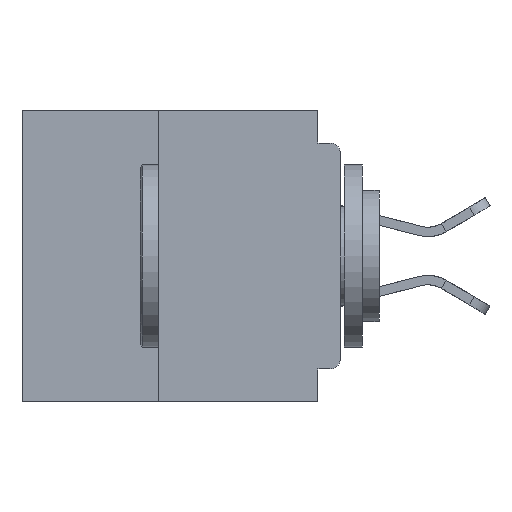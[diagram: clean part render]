
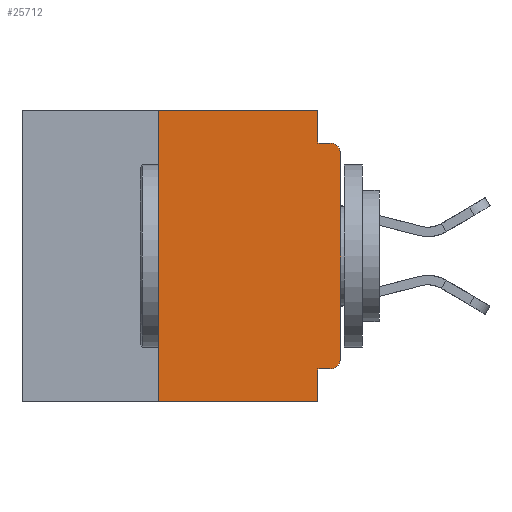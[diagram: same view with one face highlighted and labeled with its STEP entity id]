
A CAD part, left-side view. The second image highlights one B-rep face of the part: STEP entity #25712.
In plain terms, the highlighted planar face has unit normal (-1, 0, 0).
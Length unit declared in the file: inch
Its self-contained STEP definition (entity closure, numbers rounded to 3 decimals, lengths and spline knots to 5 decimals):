
#529 = DIRECTION ( 'NONE',  ( 0., 0., 1. ) ) ;
#967 = CARTESIAN_POINT ( 'NONE',  ( 0., 0.015, -0.355 ) ) ;
#1643 = VERTEX_POINT ( 'NONE', #35151 ) ;
#2192 = DIRECTION ( 'NONE',  ( 0., -1., 0. ) ) ;
#2508 = CIRCLE ( 'NONE', #37248, 0.015 ) ;
#2940 = CARTESIAN_POINT ( 'NONE',  ( 0., 0., -0.355 ) ) ;
#3272 = VECTOR ( 'NONE', #37952, 39.37008 ) ;
#4359 = VERTEX_POINT ( 'NONE', #12154 ) ;
#4495 = CARTESIAN_POINT ( 'NONE',  ( 0., 0.015, -0.34 ) ) ;
#5583 = VECTOR ( 'NONE', #36931, 39.37008 ) ;
#5776 = ORIENTED_EDGE ( 'NONE', *, *, #41378, .T. ) ;
#5811 = DIRECTION ( 'NONE',  ( 0., 0., -1. ) ) ;
#6164 = VERTEX_POINT ( 'NONE', #18352 ) ;
#6285 = LINE ( 'NONE', #29455, #47510 ) ;
#8066 = CARTESIAN_POINT ( 'NONE',  ( 0., 0.031, -0.4 ) ) ;
#8406 = DIRECTION ( 'NONE',  ( 0., 0., -1. ) ) ;
#11451 = EDGE_CURVE ( 'NONE', #26773, #46012, #16477, .T. ) ;
#11455 = AXIS2_PLACEMENT_3D ( 'NONE', #20209, #35841, #12506 ) ;
#11961 = ORIENTED_EDGE ( 'NONE', *, *, #47953, .T. ) ;
#12154 = CARTESIAN_POINT ( 'NONE',  ( 0., 0.015, -0.045 ) ) ;
#12506 = DIRECTION ( 'NONE',  ( 0., 0., -1. ) ) ;
#12715 = VECTOR ( 'NONE', #5811, 39.37008 ) ;
#13444 = EDGE_CURVE ( 'NONE', #37648, #26773, #26313, .T. ) ;
#13562 = LINE ( 'NONE', #2940, #3272 ) ;
#15649 = LINE ( 'NONE', #8066, #36321 ) ;
#16477 = LINE ( 'NONE', #44474, #46131 ) ;
#16908 = ORIENTED_EDGE ( 'NONE', *, *, #21993, .F. ) ;
#16915 = ORIENTED_EDGE ( 'NONE', *, *, #31370, .F. ) ;
#17288 = CARTESIAN_POINT ( 'NONE',  ( 0., 0.25, 0. ) ) ;
#17357 = DIRECTION ( 'NONE',  ( -1., 0., 0. ) ) ;
#18352 = CARTESIAN_POINT ( 'NONE',  ( 0., 0., -0.34 ) ) ;
#18478 = CARTESIAN_POINT ( 'NONE',  ( 0., 0.437, -0.4 ) ) ;
#20209 = CARTESIAN_POINT ( 'NONE',  ( 0., 0.437, 0. ) ) ;
#20778 = ORIENTED_EDGE ( 'NONE', *, *, #11451, .F. ) ;
#21427 = VECTOR ( 'NONE', #529, 39.37008 ) ;
#21993 = EDGE_CURVE ( 'NONE', #46012, #23897, #33446, .T. ) ;
#22427 = DIRECTION ( 'NONE',  ( 0., -1., 0. ) ) ;
#22482 = VERTEX_POINT ( 'NONE', #967 ) ;
#22801 = EDGE_CURVE ( 'NONE', #37648, #30056, #34600, .T. ) ;
#23517 = EDGE_CURVE ( 'NONE', #1643, #4359, #46537, .T. ) ;
#23897 = VERTEX_POINT ( 'NONE', #27563 ) ;
#24270 = VECTOR ( 'NONE', #22427, 39.37008 ) ;
#24434 = CARTESIAN_POINT ( 'NONE',  ( 0., 0.031, -0.355 ) ) ;
#25228 = CARTESIAN_POINT ( 'NONE',  ( 0., 0.031, 0. ) ) ;
#25274 = DIRECTION ( 'NONE',  ( 0., -1., 0. ) ) ;
#25410 = CARTESIAN_POINT ( 'NONE',  ( 0., 0.25, -0.4 ) ) ;
#25712 = ADVANCED_FACE ( 'NONE', ( #36022 ), #31965, .F. ) ;
#26313 = LINE ( 'NONE', #44622, #5583 ) ;
#26773 = VERTEX_POINT ( 'NONE', #17288 ) ;
#27563 = CARTESIAN_POINT ( 'NONE',  ( 0., 0.031, -0.045 ) ) ;
#27802 = CARTESIAN_POINT ( 'NONE',  ( 0., 0., 0. ) ) ;
#29455 = CARTESIAN_POINT ( 'NONE',  ( 0., 0., -0.045 ) ) ;
#30056 = VERTEX_POINT ( 'NONE', #31667 ) ;
#31370 = EDGE_CURVE ( 'NONE', #49707, #30056, #15649, .T. ) ;
#31377 = ORIENTED_EDGE ( 'NONE', *, *, #22801, .T. ) ;
#31667 = CARTESIAN_POINT ( 'NONE',  ( 0., 0.031, -0.4 ) ) ;
#31727 = DIRECTION ( 'NONE',  ( -1., 0., 0. ) ) ;
#31965 = PLANE ( 'NONE',  #11455 ) ;
#32606 = CARTESIAN_POINT ( 'NONE',  ( 0., 0.031, 0. ) ) ;
#33248 = AXIS2_PLACEMENT_3D ( 'NONE', #40561, #17357, #44407 ) ;
#33367 = EDGE_CURVE ( 'NONE', #22482, #49707, #13562, .T. ) ;
#33446 = LINE ( 'NONE', #25228, #12715 ) ;
#34600 = LINE ( 'NONE', #18478, #24270 ) ;
#35151 = CARTESIAN_POINT ( 'NONE',  ( 0., 0., -0.06 ) ) ;
#35253 = DIRECTION ( 'NONE',  ( 0., 0., -1. ) ) ;
#35841 = DIRECTION ( 'NONE',  ( 1., 0., 0. ) ) ;
#36022 = FACE_OUTER_BOUND ( 'NONE', #49223, .T. ) ;
#36142 = ORIENTED_EDGE ( 'NONE', *, *, #23517, .T. ) ;
#36264 = ORIENTED_EDGE ( 'NONE', *, *, #13444, .F. ) ;
#36321 = VECTOR ( 'NONE', #35253, 39.37008 ) ;
#36931 = DIRECTION ( 'NONE',  ( 0., 0., 1. ) ) ;
#37248 = AXIS2_PLACEMENT_3D ( 'NONE', #4495, #31727, #8406 ) ;
#37648 = VERTEX_POINT ( 'NONE', #25410 ) ;
#37952 = DIRECTION ( 'NONE',  ( 0., 1., 0. ) ) ;
#40561 = CARTESIAN_POINT ( 'NONE',  ( 0., 0.015, -0.06 ) ) ;
#40785 = LINE ( 'NONE', #27802, #21427 ) ;
#41378 = EDGE_CURVE ( 'NONE', #6164, #1643, #40785, .T. ) ;
#41868 = ORIENTED_EDGE ( 'NONE', *, *, #46948, .F. ) ;
#44407 = DIRECTION ( 'NONE',  ( 0., 0., -1. ) ) ;
#44474 = CARTESIAN_POINT ( 'NONE',  ( 0., 0.437, 0. ) ) ;
#44622 = CARTESIAN_POINT ( 'NONE',  ( 0., 0.25, -0.4 ) ) ;
#46012 = VERTEX_POINT ( 'NONE', #32606 ) ;
#46131 = VECTOR ( 'NONE', #25274, 39.37008 ) ;
#46537 = CIRCLE ( 'NONE', #33248, 0.015 ) ;
#46948 = EDGE_CURVE ( 'NONE', #23897, #4359, #6285, .T. ) ;
#47510 = VECTOR ( 'NONE', #2192, 39.37008 ) ;
#47953 = EDGE_CURVE ( 'NONE', #22482, #6164, #2508, .T. ) ;
#48152 = ORIENTED_EDGE ( 'NONE', *, *, #33367, .F. ) ;
#49223 = EDGE_LOOP ( 'NONE', ( #5776, #36142, #41868, #16908, #20778, #36264, #31377, #16915, #48152, #11961 ) ) ;
#49707 = VERTEX_POINT ( 'NONE', #24434 ) ;
